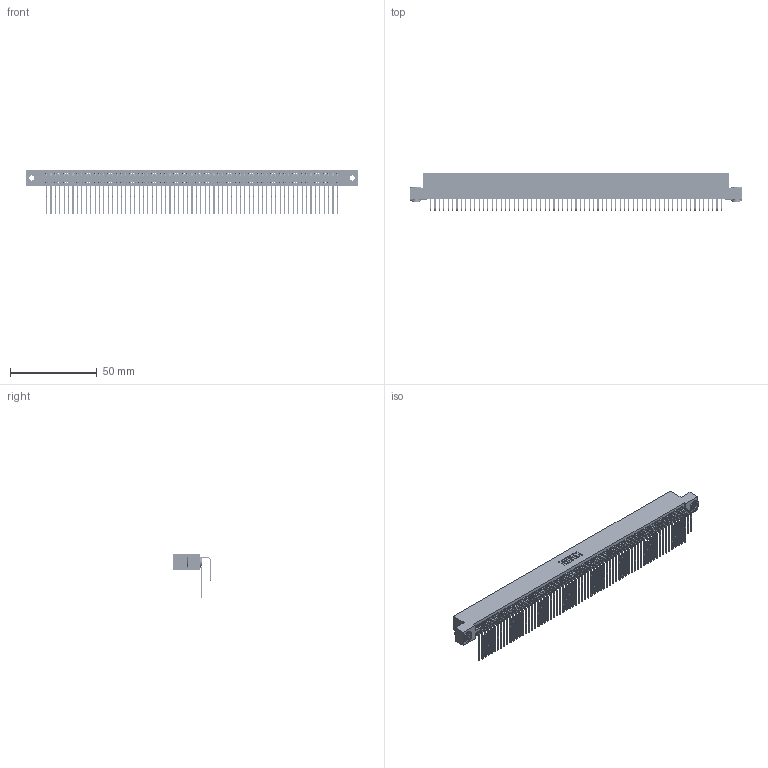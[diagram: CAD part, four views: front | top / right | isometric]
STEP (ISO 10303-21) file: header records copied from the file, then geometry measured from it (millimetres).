
FILE_DESCRIPTION (( 'STEP AP203' ), '1' );
FILE_NAME ('395-134-558-203.STEP', '2018-12-05T05:09:53', ( '' ), ( '' ), 'SwSTEP 2.0', 'SolidWorks 2016', '' );
FILE_SCHEMA (( 'CONFIG_CONTROL_DESIGN' ));
Length unit declared in the file: inch
Products named in the file (5): 395-134-558-203; 345-292-001_558 Tail - 2; 345-250-002_345-250-002-102; 345 Part_Flush Mounting Lugs - 0.156 Dia-TH; 345-292-001_558 559 Tail - 1
Assembly tree (137 placements, depth 2):
  395-134-558-203
    345 Part_Flush Mounting Lugs - 0.156 Dia-TH
    345-292-001_558 559 Tail - 1  x67
    345-292-001_558 Tail - 2  x67
    345-250-002_345-250-002-102  x2
Bounding box: 191.39 x 21.83 x 25.53 mm (x, y, z)
Volume: 19616.2 mm3; surface area: 33320.1 mm2
Topology: 137 solids, 137 shells, 7132 faces, 21187 edges, 13942 vertices
Faces by surface type: plane 4780, cylinder 2344, cone 8
Entity records: 51506 total; most frequent: CARTESIAN_POINT 8630, ORIENTED_EDGE 8506, DIRECTION 7583, EDGE_CURVE 4253, VECTOR 3789, LINE 3789, VERTEX_POINT 2830, AXIS2_PLACEMENT_3D 1897
